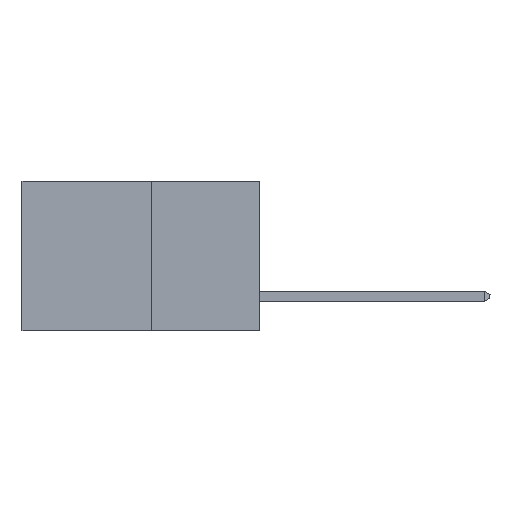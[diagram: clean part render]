
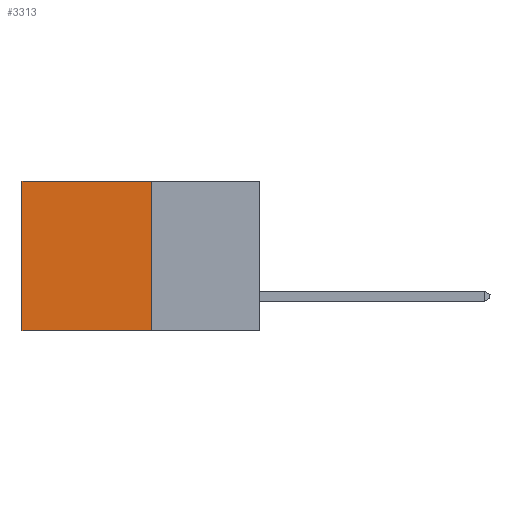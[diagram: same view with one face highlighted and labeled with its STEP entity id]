
A CAD part, left-side view. The second image highlights one B-rep face of the part: STEP entity #3313.
In plain terms, the highlighted planar face has unit normal (-1, 0, 0).
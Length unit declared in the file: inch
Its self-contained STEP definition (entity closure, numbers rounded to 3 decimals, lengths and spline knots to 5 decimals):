
#6 = VERTEX_POINT ( 'NONE', #20931 ) ;
#729 = CARTESIAN_POINT ( 'NONE',  ( 0.277, 0.27, -0.37 ) ) ;
#1160 = LINE ( 'NONE', #11325, #19277 ) ;
#1684 = EDGE_CURVE ( 'NONE', #2301, #6, #11408, .T. ) ;
#2301 = VERTEX_POINT ( 'NONE', #12329 ) ;
#3313 = ADVANCED_FACE ( 'NONE', ( #15444 ), #3493, .F. ) ;
#3427 = EDGE_LOOP ( 'NONE', ( #10484, #4728, #10821, #8015 ) ) ;
#3493 = PLANE ( 'NONE',  #12991 ) ;
#4728 = ORIENTED_EDGE ( 'NONE', *, *, #24725, .F. ) ;
#5303 = CARTESIAN_POINT ( 'NONE',  ( 0.277, 0.27, 0. ) ) ;
#6872 = DIRECTION ( 'NONE',  ( 0., 1., 0. ) ) ;
#7446 = VECTOR ( 'NONE', #6872, 39.37008 ) ;
#8015 = ORIENTED_EDGE ( 'NONE', *, *, #12558, .T. ) ;
#10484 = ORIENTED_EDGE ( 'NONE', *, *, #1684, .T. ) ;
#10768 = VECTOR ( 'NONE', #18450, 39.37008 ) ;
#10821 = ORIENTED_EDGE ( 'NONE', *, *, #18454, .F. ) ;
#11325 = CARTESIAN_POINT ( 'NONE',  ( 0.277, 0.27, -0.37 ) ) ;
#11408 = LINE ( 'NONE', #20082, #10768 ) ;
#12329 = CARTESIAN_POINT ( 'NONE',  ( 0.277, 0.59, 0. ) ) ;
#12558 = EDGE_CURVE ( 'NONE', #14303, #2301, #17627, .T. ) ;
#12984 = VECTOR ( 'NONE', #13894, 39.37008 ) ;
#12991 = AXIS2_PLACEMENT_3D ( 'NONE', #729, #16284, #13210 ) ;
#13210 = DIRECTION ( 'NONE',  ( 0., 0., -1. ) ) ;
#13704 = VERTEX_POINT ( 'NONE', #24871 ) ;
#13894 = DIRECTION ( 'NONE',  ( 0., 1., 0. ) ) ;
#14303 = VERTEX_POINT ( 'NONE', #5303 ) ;
#15417 = DIRECTION ( 'NONE',  ( 0., 0., -1. ) ) ;
#15444 = FACE_OUTER_BOUND ( 'NONE', #3427, .T. ) ;
#16284 = DIRECTION ( 'NONE',  ( 1., 0., 0. ) ) ;
#17627 = LINE ( 'NONE', #21076, #7446 ) ;
#18368 = LINE ( 'NONE', #21885, #12984 ) ;
#18450 = DIRECTION ( 'NONE',  ( 0., 0., -1. ) ) ;
#18454 = EDGE_CURVE ( 'NONE', #14303, #13704, #1160, .T. ) ;
#19277 = VECTOR ( 'NONE', #15417, 39.37008 ) ;
#20082 = CARTESIAN_POINT ( 'NONE',  ( 0.277, 0.59, -0.37 ) ) ;
#20931 = CARTESIAN_POINT ( 'NONE',  ( 0.277, 0.59, -0.37 ) ) ;
#21076 = CARTESIAN_POINT ( 'NONE',  ( 0.277, 0.27, 0. ) ) ;
#21885 = CARTESIAN_POINT ( 'NONE',  ( 0.277, 0.27, -0.37 ) ) ;
#24725 = EDGE_CURVE ( 'NONE', #13704, #6, #18368, .T. ) ;
#24871 = CARTESIAN_POINT ( 'NONE',  ( 0.277, 0.27, -0.37 ) ) ;
